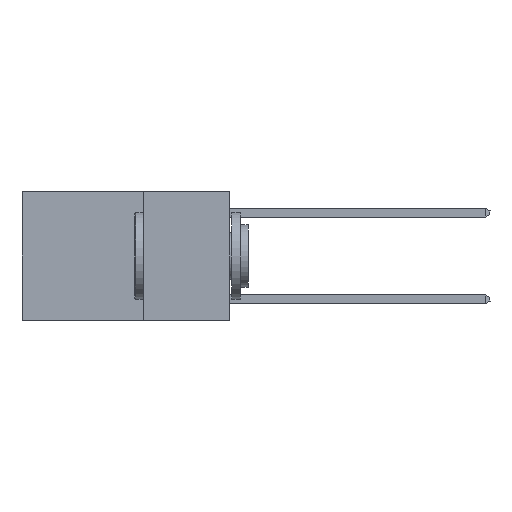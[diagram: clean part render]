
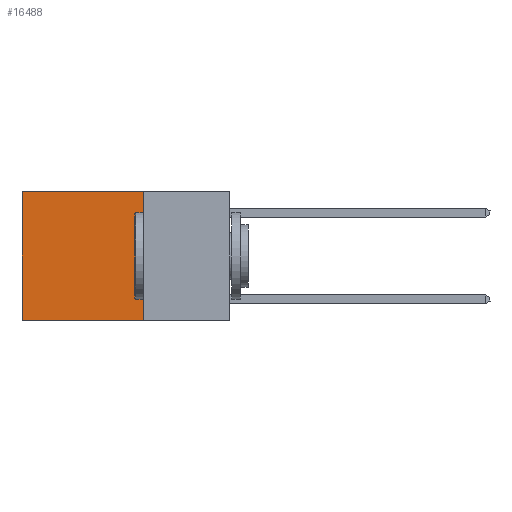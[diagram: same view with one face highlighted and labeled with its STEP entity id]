
A CAD part, left-side view. The second image highlights one B-rep face of the part: STEP entity #16488.
In plain terms, the highlighted planar face has unit normal (-1, 0, 0).
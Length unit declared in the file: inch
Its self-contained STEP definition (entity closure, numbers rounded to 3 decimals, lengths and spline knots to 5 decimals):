
#331 = VERTEX_POINT ( 'NONE', #20367 ) ;
#974 = DIRECTION ( 'NONE',  ( 0., 0., -1. ) ) ;
#1564 = EDGE_CURVE ( 'NONE', #2861, #331, #2465, .T. ) ;
#1955 = EDGE_LOOP ( 'NONE', ( #2485, #4591, #8738, #14835 ) ) ;
#2012 = FACE_OUTER_BOUND ( 'NONE', #1955, .T. ) ;
#2465 = LINE ( 'NONE', #22212, #17100 ) ;
#2485 = ORIENTED_EDGE ( 'NONE', *, *, #1564, .T. ) ;
#2565 = DIRECTION ( 'NONE',  ( 0., 0., -1. ) ) ;
#2861 = VERTEX_POINT ( 'NONE', #5528 ) ;
#3088 = VECTOR ( 'NONE', #974, 39.37008 ) ;
#3517 = DIRECTION ( 'NONE',  ( 0., 0., -1. ) ) ;
#3595 = EDGE_CURVE ( 'NONE', #6591, #331, #15260, .T. ) ;
#4432 = LINE ( 'NONE', #6634, #3088 ) ;
#4591 = ORIENTED_EDGE ( 'NONE', *, *, #3595, .F. ) ;
#5528 = CARTESIAN_POINT ( 'NONE',  ( 0.2625, 0.6, 0. ) ) ;
#5701 = VECTOR ( 'NONE', #19234, 39.37008 ) ;
#5731 = VERTEX_POINT ( 'NONE', #17261 ) ;
#6591 = VERTEX_POINT ( 'NONE', #12453 ) ;
#6634 = CARTESIAN_POINT ( 'NONE',  ( 0.2625, 0.25, 0. ) ) ;
#7240 = DIRECTION ( 'NONE',  ( 1., 0., 0. ) ) ;
#8738 = ORIENTED_EDGE ( 'NONE', *, *, #22407, .F. ) ;
#12453 = CARTESIAN_POINT ( 'NONE',  ( 0.2625, 0.25, -0.37 ) ) ;
#12899 = CARTESIAN_POINT ( 'NONE',  ( 0.2625, 0.25, 0. ) ) ;
#13888 = DIRECTION ( 'NONE',  ( 0., 1., 0. ) ) ;
#14294 = CARTESIAN_POINT ( 'NONE',  ( 0.2625, 0.25, 0. ) ) ;
#14835 = ORIENTED_EDGE ( 'NONE', *, *, #17721, .T. ) ;
#15260 = LINE ( 'NONE', #22317, #16439 ) ;
#15316 = LINE ( 'NONE', #14294, #5701 ) ;
#16327 = AXIS2_PLACEMENT_3D ( 'NONE', #12899, #7240, #3517 ) ;
#16439 = VECTOR ( 'NONE', #13888, 39.37008 ) ;
#16488 = ADVANCED_FACE ( 'NONE', ( #2012 ), #19586, .F. ) ;
#17100 = VECTOR ( 'NONE', #2565, 39.37008 ) ;
#17261 = CARTESIAN_POINT ( 'NONE',  ( 0.2625, 0.25, 0. ) ) ;
#17721 = EDGE_CURVE ( 'NONE', #5731, #2861, #15316, .T. ) ;
#19234 = DIRECTION ( 'NONE',  ( 0., 1., 0. ) ) ;
#19586 = PLANE ( 'NONE',  #16327 ) ;
#20367 = CARTESIAN_POINT ( 'NONE',  ( 0.2625, 0.6, -0.37 ) ) ;
#22212 = CARTESIAN_POINT ( 'NONE',  ( 0.2625, 0.6, 0. ) ) ;
#22317 = CARTESIAN_POINT ( 'NONE',  ( 0.2625, 0.25, -0.37 ) ) ;
#22407 = EDGE_CURVE ( 'NONE', #5731, #6591, #4432, .T. ) ;
